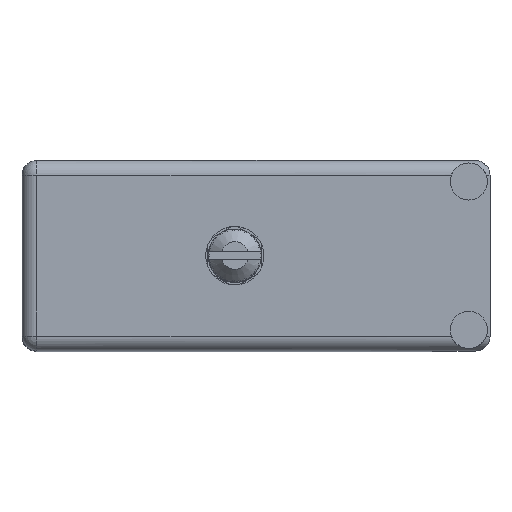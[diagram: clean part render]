
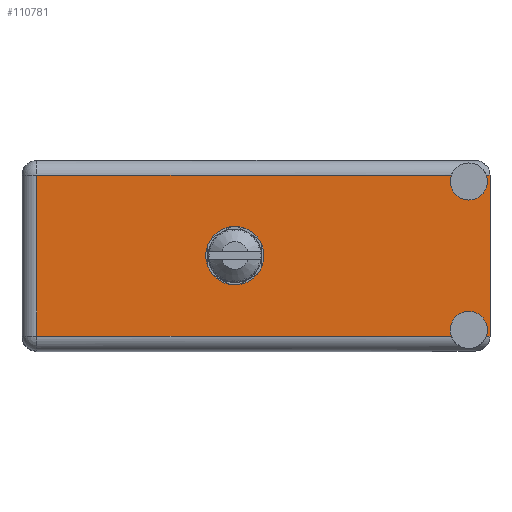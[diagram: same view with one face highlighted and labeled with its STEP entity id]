
A CAD part, top view. The second image highlights one B-rep face of the part: STEP entity #110781.
In plain terms, the highlighted face is planar.
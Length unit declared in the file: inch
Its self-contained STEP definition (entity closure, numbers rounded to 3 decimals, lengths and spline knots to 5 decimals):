
#847 = AXIS2_PLACEMENT_3D ( 'NONE', #85386, #17637, #9585 ) ;
#5441 = LINE ( 'NONE', #11341, #76549 ) ;
#5690 = ORIENTED_EDGE ( 'NONE', *, *, #108226, .F. ) ;
#7961 = CIRCLE ( 'NONE', #847, 0.1375 ) ;
#8343 = ORIENTED_EDGE ( 'NONE', *, *, #91442, .T. ) ;
#8368 = CARTESIAN_POINT ( 'NONE',  ( 1.004, 1.566, -0.4495 ) ) ;
#8491 = VECTOR ( 'NONE', #15120, 39.37008 ) ;
#9585 = DIRECTION ( 'NONE',  ( 0., 0., 1. ) ) ;
#9663 = LINE ( 'NONE', #21952, #76708 ) ;
#11341 = CARTESIAN_POINT ( 'NONE',  ( 0.07, 1.566, -0.899 ) ) ;
#13093 = FACE_OUTER_BOUND ( 'NONE', #112190, .T. ) ;
#15120 = DIRECTION ( 'NONE',  ( -1., 0., 0. ) ) ;
#15473 = DIRECTION ( 'NONE',  ( 0., 0., 1. ) ) ;
#15646 = CIRCLE ( 'NONE', #33682, 0.0875 ) ;
#15877 = CARTESIAN_POINT ( 'NONE',  ( 2.19038, 1.566, -0.07 ) ) ;
#16768 = CARTESIAN_POINT ( 'NONE',  ( 2.108, 1.566, -0.7995 ) ) ;
#16991 = CARTESIAN_POINT ( 'NONE',  ( 2.108, 1.566, -0.0995 ) ) ;
#17637 = DIRECTION ( 'NONE',  ( 0., 1., 0. ) ) ;
#21952 = CARTESIAN_POINT ( 'NONE',  ( 0., 1.566, -0.829 ) ) ;
#23341 = VERTEX_POINT ( 'NONE', #49953 ) ;
#23409 = CARTESIAN_POINT ( 'NONE',  ( 0.07, 1.566, -0.829 ) ) ;
#23748 = DIRECTION ( 'NONE',  ( 0., 1., 0. ) ) ;
#24009 = ORIENTED_EDGE ( 'NONE', *, *, #99524, .T. ) ;
#24383 = VERTEX_POINT ( 'NONE', #93670 ) ;
#25611 = DIRECTION ( 'NONE',  ( 0., 1., 0. ) ) ;
#25793 = CIRCLE ( 'NONE', #84086, 0.0875 ) ;
#25914 = LINE ( 'NONE', #66366, #50543 ) ;
#26949 = AXIS2_PLACEMENT_3D ( 'NONE', #95243, #59597, #86392 ) ;
#27678 = EDGE_CURVE ( 'NONE', #23341, #66758, #42849, .T. ) ;
#28427 = AXIS2_PLACEMENT_3D ( 'NONE', #28806, #63994, #108148 ) ;
#28806 = CARTESIAN_POINT ( 'NONE',  ( 2.108, 1.566, -0.7995 ) ) ;
#30242 = VERTEX_POINT ( 'NONE', #65128 ) ;
#31195 = EDGE_LOOP ( 'NONE', ( #5690, #96575 ) ) ;
#33040 = CARTESIAN_POINT ( 'NONE',  ( 1.004, 1.566, -0.312 ) ) ;
#33682 = AXIS2_PLACEMENT_3D ( 'NONE', #16991, #68684, #15473 ) ;
#34009 = PLANE ( 'NONE',  #26949 ) ;
#35937 = VERTEX_POINT ( 'NONE', #52776 ) ;
#39622 = VERTEX_POINT ( 'NONE', #23409 ) ;
#42040 = CARTESIAN_POINT ( 'NONE',  ( 2.208, 1.566, -0.07 ) ) ;
#42849 = LINE ( 'NONE', #58397, #8491 ) ;
#44184 = ORIENTED_EDGE ( 'NONE', *, *, #27678, .T. ) ;
#44212 = CARTESIAN_POINT ( 'NONE',  ( 2.208, 1.566, -0.07 ) ) ;
#45259 = CIRCLE ( 'NONE', #73943, 0.0875 ) ;
#47353 = LINE ( 'NONE', #42040, #50088 ) ;
#49953 = CARTESIAN_POINT ( 'NONE',  ( 2.208, 1.566, -0.829 ) ) ;
#50088 = VECTOR ( 'NONE', #103307, 39.37008 ) ;
#50543 = VECTOR ( 'NONE', #68658, 39.37008 ) ;
#52601 = CIRCLE ( 'NONE', #86745, 0.1375 ) ;
#52776 = CARTESIAN_POINT ( 'NONE',  ( 2.02562, 1.566, -0.07 ) ) ;
#52811 = DIRECTION ( 'NONE',  ( 0., 0., 1. ) ) ;
#54445 = EDGE_CURVE ( 'NONE', #23341, #58067, #25914, .T. ) ;
#55781 = CARTESIAN_POINT ( 'NONE',  ( 2.208, 1.566, -0.07 ) ) ;
#58067 = VERTEX_POINT ( 'NONE', #44212 ) ;
#58397 = CARTESIAN_POINT ( 'NONE',  ( 0., 1.566, -0.829 ) ) ;
#58959 = VERTEX_POINT ( 'NONE', #15877 ) ;
#59597 = DIRECTION ( 'NONE',  ( 0., 1., 0. ) ) ;
#60492 = ORIENTED_EDGE ( 'NONE', *, *, #111757, .F. ) ;
#63994 = DIRECTION ( 'NONE',  ( 0., 1., 0. ) ) ;
#64277 = CARTESIAN_POINT ( 'NONE',  ( 2.108, 1.566, -0.712 ) ) ;
#65128 = CARTESIAN_POINT ( 'NONE',  ( 0.07, 1.566, -0.07 ) ) ;
#65169 = ORIENTED_EDGE ( 'NONE', *, *, #112363, .F. ) ;
#66366 = CARTESIAN_POINT ( 'NONE',  ( 2.208, 1.566, 0. ) ) ;
#66758 = VERTEX_POINT ( 'NONE', #83761 ) ;
#67738 = DIRECTION ( 'NONE',  ( 0., 0., 1. ) ) ;
#67888 = ORIENTED_EDGE ( 'NONE', *, *, #102315, .T. ) ;
#68658 = DIRECTION ( 'NONE',  ( 0., 0., 1. ) ) ;
#68684 = DIRECTION ( 'NONE',  ( 0., 1., 0. ) ) ;
#71447 = EDGE_CURVE ( 'NONE', #58959, #58067, #47353, .T. ) ;
#72366 = EDGE_CURVE ( 'NONE', #24383, #92395, #52601, .T. ) ;
#73943 = AXIS2_PLACEMENT_3D ( 'NONE', #16768, #25611, #111819 ) ;
#75579 = DIRECTION ( 'NONE',  ( 1., 0., 0. ) ) ;
#76094 = CARTESIAN_POINT ( 'NONE',  ( 2.108, 1.566, -0.0995 ) ) ;
#76549 = VECTOR ( 'NONE', #91327, 39.37008 ) ;
#76708 = VECTOR ( 'NONE', #92414, 39.37008 ) ;
#79984 = ORIENTED_EDGE ( 'NONE', *, *, #100540, .F. ) ;
#81618 = FACE_BOUND ( 'NONE', #31195, .T. ) ;
#82248 = CARTESIAN_POINT ( 'NONE',  ( 2.108, 1.566, -0.187 ) ) ;
#82505 = VERTEX_POINT ( 'NONE', #100947 ) ;
#83390 = VERTEX_POINT ( 'NONE', #82248 ) ;
#83761 = CARTESIAN_POINT ( 'NONE',  ( 2.19038, 1.566, -0.829 ) ) ;
#83874 = VERTEX_POINT ( 'NONE', #64277 ) ;
#84086 = AXIS2_PLACEMENT_3D ( 'NONE', #76094, #23748, #67738 ) ;
#85386 = CARTESIAN_POINT ( 'NONE',  ( 1.004, 1.566, -0.4495 ) ) ;
#86392 = DIRECTION ( 'NONE',  ( 0., 0., 1. ) ) ;
#86745 = AXIS2_PLACEMENT_3D ( 'NONE', #8368, #104917, #52811 ) ;
#88634 = VECTOR ( 'NONE', #75579, 39.37008 ) ;
#88835 = ORIENTED_EDGE ( 'NONE', *, *, #54445, .F. ) ;
#91327 = DIRECTION ( 'NONE',  ( 0., 0., 1. ) ) ;
#91442 = EDGE_CURVE ( 'NONE', #82505, #39622, #9663, .T. ) ;
#92395 = VERTEX_POINT ( 'NONE', #33040 ) ;
#92414 = DIRECTION ( 'NONE',  ( -1., 0., 0. ) ) ;
#93670 = CARTESIAN_POINT ( 'NONE',  ( 1.004, 1.566, -0.587 ) ) ;
#95243 = CARTESIAN_POINT ( 'NONE',  ( 0., 1.566, -0.899 ) ) ;
#96575 = ORIENTED_EDGE ( 'NONE', *, *, #72366, .F. ) ;
#99403 = ORIENTED_EDGE ( 'NONE', *, *, #106244, .F. ) ;
#99524 = EDGE_CURVE ( 'NONE', #39622, #30242, #5441, .T. ) ;
#100540 = EDGE_CURVE ( 'NONE', #58959, #83390, #25793, .T. ) ;
#100947 = CARTESIAN_POINT ( 'NONE',  ( 2.02562, 1.566, -0.829 ) ) ;
#100949 = LINE ( 'NONE', #55781, #88634 ) ;
#102315 = EDGE_CURVE ( 'NONE', #30242, #35937, #100949, .T. ) ;
#103307 = DIRECTION ( 'NONE',  ( 1., 0., 0. ) ) ;
#104844 = CIRCLE ( 'NONE', #28427, 0.0875 ) ;
#104917 = DIRECTION ( 'NONE',  ( 0., 1., 0. ) ) ;
#105479 = ORIENTED_EDGE ( 'NONE', *, *, #71447, .T. ) ;
#106244 = EDGE_CURVE ( 'NONE', #83874, #66758, #45259, .T. ) ;
#108148 = DIRECTION ( 'NONE',  ( 0., 0., 1. ) ) ;
#108226 = EDGE_CURVE ( 'NONE', #92395, #24383, #7961, .T. ) ;
#110781 = ADVANCED_FACE ( 'NONE', ( #81618, #13093 ), #34009, .T. ) ;
#111757 = EDGE_CURVE ( 'NONE', #82505, #83874, #104844, .T. ) ;
#111819 = DIRECTION ( 'NONE',  ( 0., 0., 1. ) ) ;
#112190 = EDGE_LOOP ( 'NONE', ( #67888, #65169, #79984, #105479, #88835, #44184, #99403, #60492, #8343, #24009 ) ) ;
#112363 = EDGE_CURVE ( 'NONE', #83390, #35937, #15646, .T. ) ;
